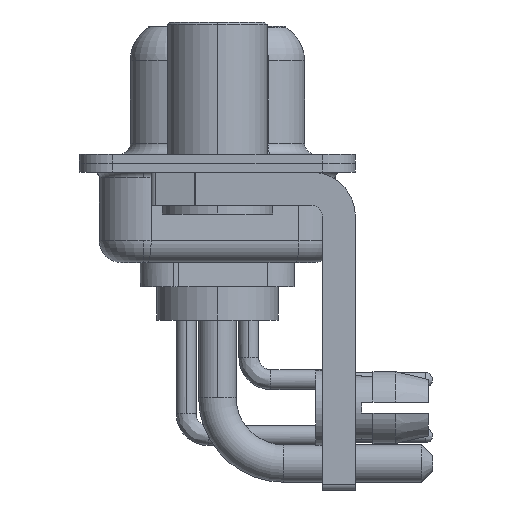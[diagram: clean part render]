
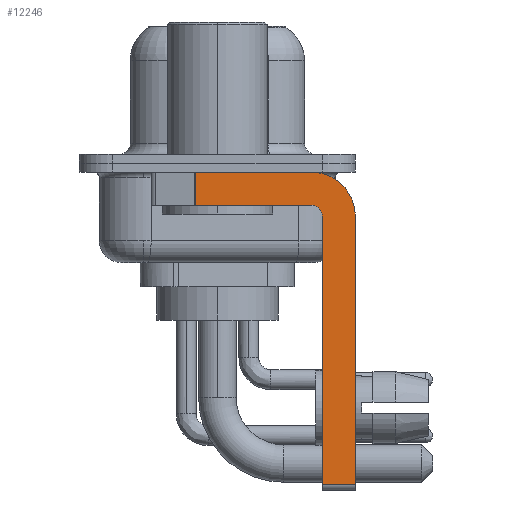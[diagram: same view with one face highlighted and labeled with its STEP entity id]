
A CAD part, left-side view. The second image highlights one B-rep face of the part: STEP entity #12246.
In plain terms, the highlighted planar face has unit normal (-1, 0, 0).
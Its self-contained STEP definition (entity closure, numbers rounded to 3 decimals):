
#471 = VERTEX_POINT ( 'NONE', #12535 ) ;
#837 = DIRECTION ( 'NONE',  ( 0., -1., 0. ) ) ;
#1102 = CARTESIAN_POINT ( 'NONE',  ( -2.9, -4.75, -2.4 ) ) ;
#1652 = CARTESIAN_POINT ( 'NONE',  ( -2.9, -4.75, -14.8 ) ) ;
#1992 = DIRECTION ( 'NONE',  ( 0., 0., -1. ) ) ;
#2300 = LINE ( 'NONE', #18201, #10255 ) ;
#2578 = VECTOR ( 'NONE', #5104, 1000. ) ;
#3261 = AXIS2_PLACEMENT_3D ( 'NONE', #11365, #3849, #11763 ) ;
#3316 = LINE ( 'NONE', #1652, #7571 ) ;
#3651 = VERTEX_POINT ( 'NONE', #4206 ) ;
#3849 = DIRECTION ( 'NONE',  ( 1., 0., 0. ) ) ;
#3866 = EDGE_CURVE ( 'NONE', #3651, #18809, #17770, .T. ) ;
#4206 = CARTESIAN_POINT ( 'NONE',  ( -2.9, 0.978, -0.4 ) ) ;
#4373 = LINE ( 'NONE', #20587, #5976 ) ;
#4529 = DIRECTION ( 'NONE',  ( 0., 0., -1. ) ) ;
#5101 = ORIENTED_EDGE ( 'NONE', *, *, #8004, .F. ) ;
#5104 = DIRECTION ( 'NONE',  ( 0., 1., 0. ) ) ;
#5148 = ORIENTED_EDGE ( 'NONE', *, *, #5918, .F. ) ;
#5211 = CARTESIAN_POINT ( 'NONE',  ( -2.9, -4.25, -1.9 ) ) ;
#5495 = EDGE_CURVE ( 'NONE', #20383, #15273, #2300, .T. ) ;
#5896 = CARTESIAN_POINT ( 'NONE',  ( -2.9, -4.25, -2.4 ) ) ;
#5918 = EDGE_CURVE ( 'NONE', #9896, #9574, #3316, .T. ) ;
#5956 = CIRCLE ( 'NONE', #12351, 2. ) ;
#5976 = VECTOR ( 'NONE', #13865, 1000. ) ;
#6218 = EDGE_LOOP ( 'NONE', ( #17001, #18667, #5101, #17426, #5148, #13345, #11476, #11080 ) ) ;
#6738 = VERTEX_POINT ( 'NONE', #16856 ) ;
#7571 = VECTOR ( 'NONE', #15764, 1000. ) ;
#7606 = EDGE_CURVE ( 'NONE', #6738, #20383, #5956, .T. ) ;
#7807 = EDGE_CURVE ( 'NONE', #9896, #15273, #4373, .T. ) ;
#8004 = EDGE_CURVE ( 'NONE', #471, #18809, #14473, .T. ) ;
#8009 = CIRCLE ( 'NONE', #10704, 0.5 ) ;
#8714 = DIRECTION ( 'NONE',  ( 0., 0., -1. ) ) ;
#8848 = LINE ( 'NONE', #18209, #16447 ) ;
#9223 = CARTESIAN_POINT ( 'NONE',  ( -2.9, 0.978, -1.9 ) ) ;
#9574 = VERTEX_POINT ( 'NONE', #1102 ) ;
#9896 = VERTEX_POINT ( 'NONE', #18649 ) ;
#9981 = CARTESIAN_POINT ( 'NONE',  ( -2.9, -4.25, -2.4 ) ) ;
#10255 = VECTOR ( 'NONE', #1992, 1000. ) ;
#10704 = AXIS2_PLACEMENT_3D ( 'NONE', #5896, #12326, #15576 ) ;
#11080 = ORIENTED_EDGE ( 'NONE', *, *, #7606, .F. ) ;
#11365 = CARTESIAN_POINT ( 'NONE',  ( -2.9, -4.25, -2.4 ) ) ;
#11476 = ORIENTED_EDGE ( 'NONE', *, *, #5495, .F. ) ;
#11763 = DIRECTION ( 'NONE',  ( 0., 0., -1. ) ) ;
#11827 = CARTESIAN_POINT ( 'NONE',  ( -2.9, -6.25, -2.4 ) ) ;
#12155 = EDGE_CURVE ( 'NONE', #9574, #471, #8009, .T. ) ;
#12246 = ADVANCED_FACE ( 'NONE', ( #13323 ), #14408, .F. ) ;
#12326 = DIRECTION ( 'NONE',  ( -1., 0., 0. ) ) ;
#12351 = AXIS2_PLACEMENT_3D ( 'NONE', #9981, #14806, #8714 ) ;
#12535 = CARTESIAN_POINT ( 'NONE',  ( -2.9, -4.25, -1.9 ) ) ;
#13323 = FACE_OUTER_BOUND ( 'NONE', #6218, .T. ) ;
#13345 = ORIENTED_EDGE ( 'NONE', *, *, #7807, .T. ) ;
#13499 = VECTOR ( 'NONE', #4529, 1000. ) ;
#13865 = DIRECTION ( 'NONE',  ( 0., -1., 0. ) ) ;
#14212 = CARTESIAN_POINT ( 'NONE',  ( -2.9, 0.978, -1.9 ) ) ;
#14408 = PLANE ( 'NONE',  #3261 ) ;
#14473 = LINE ( 'NONE', #5211, #2578 ) ;
#14806 = DIRECTION ( 'NONE',  ( 1., 0., 0. ) ) ;
#15190 = EDGE_CURVE ( 'NONE', #3651, #6738, #8848, .T. ) ;
#15273 = VERTEX_POINT ( 'NONE', #18839 ) ;
#15576 = DIRECTION ( 'NONE',  ( 0., 0., 1. ) ) ;
#15764 = DIRECTION ( 'NONE',  ( 0., 0., 1. ) ) ;
#16447 = VECTOR ( 'NONE', #837, 1000. ) ;
#16856 = CARTESIAN_POINT ( 'NONE',  ( -2.9, -4.25, -0.4 ) ) ;
#17001 = ORIENTED_EDGE ( 'NONE', *, *, #15190, .F. ) ;
#17426 = ORIENTED_EDGE ( 'NONE', *, *, #12155, .F. ) ;
#17770 = LINE ( 'NONE', #14212, #13499 ) ;
#18201 = CARTESIAN_POINT ( 'NONE',  ( -2.9, -6.25, -2.4 ) ) ;
#18209 = CARTESIAN_POINT ( 'NONE',  ( -2.9, 3., -0.4 ) ) ;
#18649 = CARTESIAN_POINT ( 'NONE',  ( -2.9, -4.75, -14.55 ) ) ;
#18667 = ORIENTED_EDGE ( 'NONE', *, *, #3866, .T. ) ;
#18809 = VERTEX_POINT ( 'NONE', #9223 ) ;
#18839 = CARTESIAN_POINT ( 'NONE',  ( -2.9, -6.25, -14.55 ) ) ;
#20383 = VERTEX_POINT ( 'NONE', #11827 ) ;
#20587 = CARTESIAN_POINT ( 'NONE',  ( -2.9, -4.25, -14.55 ) ) ;
